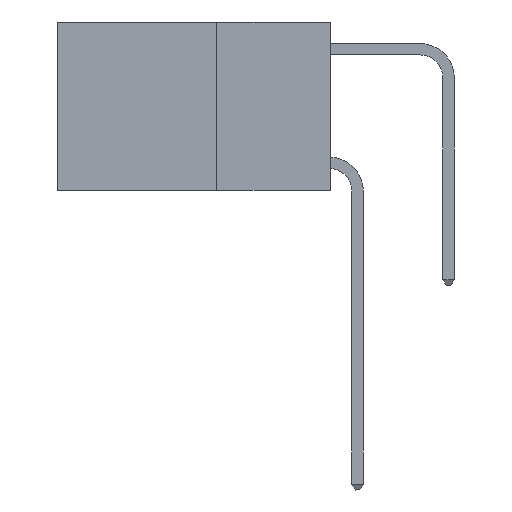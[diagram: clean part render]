
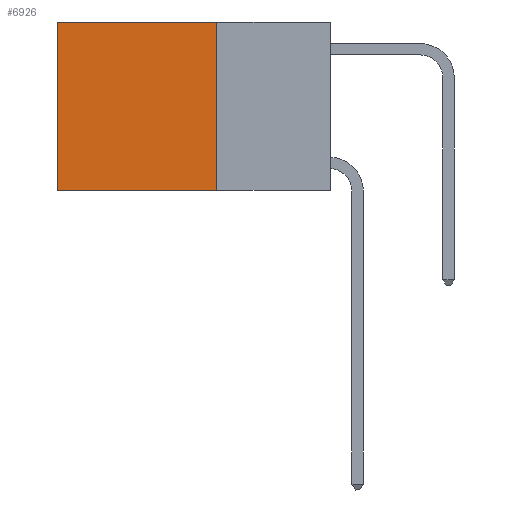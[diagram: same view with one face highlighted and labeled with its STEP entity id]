
A CAD part, left-side view. The second image highlights one B-rep face of the part: STEP entity #6926.
In plain terms, the highlighted planar face has unit normal (-1, 0, 0).
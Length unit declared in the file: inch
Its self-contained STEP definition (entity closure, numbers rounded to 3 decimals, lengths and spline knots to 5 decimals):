
#298 = CARTESIAN_POINT ( 'NONE',  ( 0.2625, 0.6, 0. ) ) ;
#476 = DIRECTION ( 'NONE',  ( 0., 0., -1. ) ) ;
#500 = DIRECTION ( 'NONE',  ( 1., 0., 0. ) ) ;
#580 = CARTESIAN_POINT ( 'NONE',  ( 0.2625, 0.25, 0. ) ) ;
#586 = PLANE ( 'NONE',  #6534 ) ;
#1286 = VECTOR ( 'NONE', #5726, 39.37008 ) ;
#1330 = VERTEX_POINT ( 'NONE', #4596 ) ;
#1575 = LINE ( 'NONE', #7348, #1286 ) ;
#1977 = EDGE_CURVE ( 'NONE', #7197, #3714, #10750, .T. ) ;
#2036 = CARTESIAN_POINT ( 'NONE',  ( 0.2625, 0.25, 0. ) ) ;
#2483 = FACE_OUTER_BOUND ( 'NONE', #6566, .T. ) ;
#2679 = DIRECTION ( 'NONE',  ( 0., 0., -1. ) ) ;
#2711 = ORIENTED_EDGE ( 'NONE', *, *, #10638, .F. ) ;
#2763 = ORIENTED_EDGE ( 'NONE', *, *, #2783, .T. ) ;
#2777 = ORIENTED_EDGE ( 'NONE', *, *, #1977, .T. ) ;
#2783 = EDGE_CURVE ( 'NONE', #3714, #9585, #10128, .T. ) ;
#2784 = ORIENTED_EDGE ( 'NONE', *, *, #9251, .F. ) ;
#3529 = VECTOR ( 'NONE', #2679, 39.37008 ) ;
#3577 = CARTESIAN_POINT ( 'NONE',  ( 0.2625, 0.25, -0.37 ) ) ;
#3594 = VECTOR ( 'NONE', #9405, 39.37008 ) ;
#3714 = VERTEX_POINT ( 'NONE', #8856 ) ;
#3857 = CARTESIAN_POINT ( 'NONE',  ( 0.2625, 0.25, 0. ) ) ;
#4596 = CARTESIAN_POINT ( 'NONE',  ( 0.2625, 0.25, -0.37 ) ) ;
#5298 = CARTESIAN_POINT ( 'NONE',  ( 0.2625, 0.6, -0.37 ) ) ;
#5726 = DIRECTION ( 'NONE',  ( 0., 0., -1. ) ) ;
#6534 = AXIS2_PLACEMENT_3D ( 'NONE', #580, #500, #476 ) ;
#6566 = EDGE_LOOP ( 'NONE', ( #2763, #2711, #2784, #2777 ) ) ;
#6733 = DIRECTION ( 'NONE',  ( 0., 1., 0. ) ) ;
#6926 = ADVANCED_FACE ( 'NONE', ( #2483 ), #586, .F. ) ;
#7197 = VERTEX_POINT ( 'NONE', #2036 ) ;
#7348 = CARTESIAN_POINT ( 'NONE',  ( 0.2625, 0.25, 0. ) ) ;
#7791 = LINE ( 'NONE', #3577, #3594 ) ;
#8636 = VECTOR ( 'NONE', #6733, 39.37008 ) ;
#8856 = CARTESIAN_POINT ( 'NONE',  ( 0.2625, 0.6, 0. ) ) ;
#9251 = EDGE_CURVE ( 'NONE', #7197, #1330, #1575, .T. ) ;
#9405 = DIRECTION ( 'NONE',  ( 0., 1., 0. ) ) ;
#9585 = VERTEX_POINT ( 'NONE', #5298 ) ;
#10128 = LINE ( 'NONE', #298, #3529 ) ;
#10638 = EDGE_CURVE ( 'NONE', #1330, #9585, #7791, .T. ) ;
#10750 = LINE ( 'NONE', #3857, #8636 ) ;
